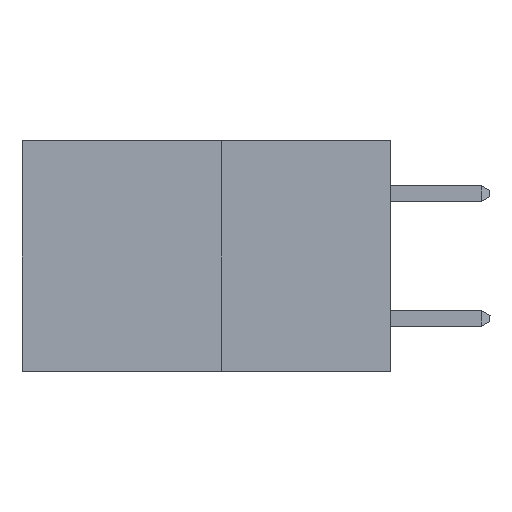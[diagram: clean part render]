
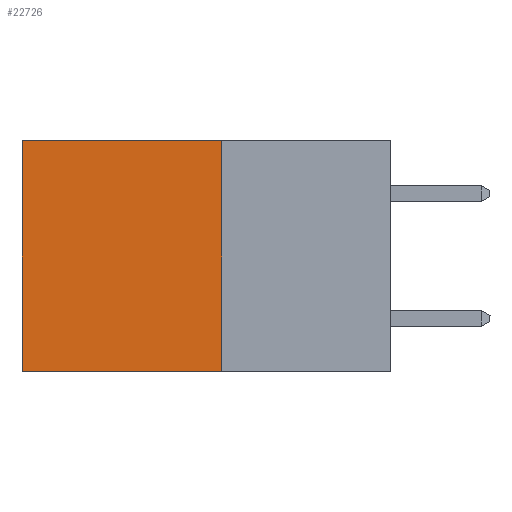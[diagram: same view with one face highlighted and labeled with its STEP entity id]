
A CAD part, left-side view. The second image highlights one B-rep face of the part: STEP entity #22726.
In plain terms, the highlighted planar face has unit normal (-1, 0, 0).
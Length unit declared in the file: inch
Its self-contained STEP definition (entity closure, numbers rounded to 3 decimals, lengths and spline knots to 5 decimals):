
#689 = DIRECTION ( 'NONE',  ( 1., 0., 0. ) ) ;
#1059 = VECTOR ( 'NONE', #11008, 39.37008 ) ;
#2832 = EDGE_LOOP ( 'NONE', ( #15424, #21006, #16588, #12261 ) ) ;
#3155 = EDGE_CURVE ( 'NONE', #4540, #10943, #16606, .T. ) ;
#4540 = VERTEX_POINT ( 'NONE', #14271 ) ;
#4567 = VERTEX_POINT ( 'NONE', #13881 ) ;
#5177 = DIRECTION ( 'NONE',  ( 0., 0., -1. ) ) ;
#5448 = CARTESIAN_POINT ( 'NONE',  ( 0.277, 0.27, -0.37 ) ) ;
#5449 = VECTOR ( 'NONE', #5177, 39.37008 ) ;
#6174 = FACE_OUTER_BOUND ( 'NONE', #2832, .T. ) ;
#8047 = VECTOR ( 'NONE', #24165, 39.37008 ) ;
#8945 = CARTESIAN_POINT ( 'NONE',  ( 0.277, 0.59, -0.37 ) ) ;
#9025 = CARTESIAN_POINT ( 'NONE',  ( 0.277, 0.59, -0.37 ) ) ;
#9029 = CARTESIAN_POINT ( 'NONE',  ( 0.277, 0.27, -0.37 ) ) ;
#10943 = VERTEX_POINT ( 'NONE', #21176 ) ;
#11008 = DIRECTION ( 'NONE',  ( 0., 0., -1. ) ) ;
#12118 = CARTESIAN_POINT ( 'NONE',  ( 0.277, 0.27, -0.37 ) ) ;
#12261 = ORIENTED_EDGE ( 'NONE', *, *, #23065, .T. ) ;
#13092 = LINE ( 'NONE', #5448, #8047 ) ;
#13570 = LINE ( 'NONE', #17589, #22880 ) ;
#13881 = CARTESIAN_POINT ( 'NONE',  ( 0.277, 0.59, 0. ) ) ;
#13978 = DIRECTION ( 'NONE',  ( 0., 0., -1. ) ) ;
#13982 = VERTEX_POINT ( 'NONE', #8945 ) ;
#14271 = CARTESIAN_POINT ( 'NONE',  ( 0.277, 0.27, 0. ) ) ;
#15424 = ORIENTED_EDGE ( 'NONE', *, *, #18857, .T. ) ;
#16143 = LINE ( 'NONE', #9025, #1059 ) ;
#16588 = ORIENTED_EDGE ( 'NONE', *, *, #3155, .F. ) ;
#16606 = LINE ( 'NONE', #9029, #5449 ) ;
#16972 = EDGE_CURVE ( 'NONE', #10943, #13982, #13092, .T. ) ;
#17589 = CARTESIAN_POINT ( 'NONE',  ( 0.277, 0.27, 0. ) ) ;
#18857 = EDGE_CURVE ( 'NONE', #4567, #13982, #16143, .T. ) ;
#19500 = DIRECTION ( 'NONE',  ( 0., 1., 0. ) ) ;
#20481 = AXIS2_PLACEMENT_3D ( 'NONE', #12118, #689, #13978 ) ;
#21006 = ORIENTED_EDGE ( 'NONE', *, *, #16972, .F. ) ;
#21176 = CARTESIAN_POINT ( 'NONE',  ( 0.277, 0.27, -0.37 ) ) ;
#21414 = PLANE ( 'NONE',  #20481 ) ;
#22726 = ADVANCED_FACE ( 'NONE', ( #6174 ), #21414, .F. ) ;
#22880 = VECTOR ( 'NONE', #19500, 39.37008 ) ;
#23065 = EDGE_CURVE ( 'NONE', #4540, #4567, #13570, .T. ) ;
#24165 = DIRECTION ( 'NONE',  ( 0., 1., 0. ) ) ;
